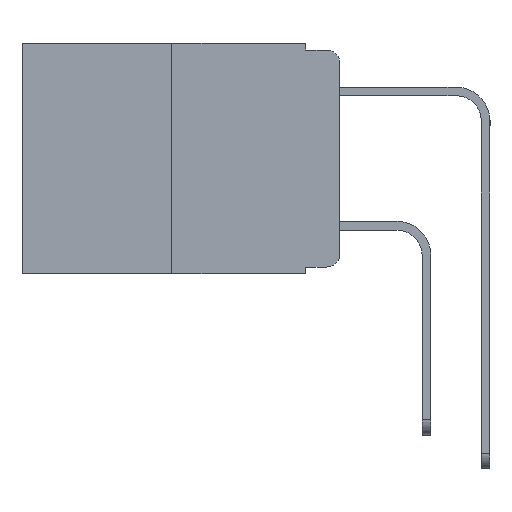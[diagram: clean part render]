
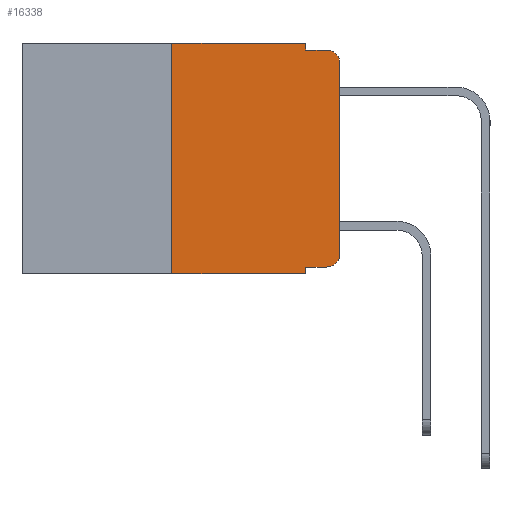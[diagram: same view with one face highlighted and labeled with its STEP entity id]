
A CAD part, left-side view. The second image highlights one B-rep face of the part: STEP entity #16338.
In plain terms, the highlighted planar face has unit normal (-1, 0, 0).
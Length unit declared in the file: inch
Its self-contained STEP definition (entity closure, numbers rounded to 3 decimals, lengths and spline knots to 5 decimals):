
#49 = DIRECTION ( 'NONE',  ( 0., 0., 1. ) ) ;
#77 = CARTESIAN_POINT ( 'NONE',  ( 0., 0.473, 0. ) ) ;
#193 = VERTEX_POINT ( 'NONE', #14427 ) ;
#359 = EDGE_CURVE ( 'NONE', #5972, #6519, #20675, .T. ) ;
#773 = LINE ( 'NONE', #20792, #4306 ) ;
#955 = DIRECTION ( 'NONE',  ( 0., -1., 0. ) ) ;
#1421 = VERTEX_POINT ( 'NONE', #14616 ) ;
#1501 = CARTESIAN_POINT ( 'NONE',  ( 0., 0.02, -0.333 ) ) ;
#1527 = DIRECTION ( 'NONE',  ( -1., 0., 0. ) ) ;
#1548 = EDGE_CURVE ( 'NONE', #13348, #5972, #15921, .T. ) ;
#1756 = DIRECTION ( 'NONE',  ( 0., -1., 0. ) ) ;
#2009 = LINE ( 'NONE', #14542, #18896 ) ;
#2579 = DIRECTION ( 'NONE',  ( 0., 0., 1. ) ) ;
#2585 = CARTESIAN_POINT ( 'NONE',  ( 0., 0., -0.313 ) ) ;
#2716 = EDGE_CURVE ( 'NONE', #13348, #1421, #773, .T. ) ;
#3867 = EDGE_CURVE ( 'NONE', #18301, #6863, #8539, .T. ) ;
#4006 = VECTOR ( 'NONE', #49, 39.37008 ) ;
#4306 = VECTOR ( 'NONE', #13086, 39.37008 ) ;
#4534 = ORIENTED_EDGE ( 'NONE', *, *, #4931, .F. ) ;
#4762 = DIRECTION ( 'NONE',  ( 1., 0., 0. ) ) ;
#4931 = EDGE_CURVE ( 'NONE', #6863, #7960, #19142, .T. ) ;
#5058 = ORIENTED_EDGE ( 'NONE', *, *, #7313, .T. ) ;
#5076 = EDGE_CURVE ( 'NONE', #7960, #16210, #2009, .T. ) ;
#5972 = VERTEX_POINT ( 'NONE', #1501 ) ;
#6217 = EDGE_CURVE ( 'NONE', #16210, #6325, #12436, .T. ) ;
#6325 = VERTEX_POINT ( 'NONE', #10806 ) ;
#6481 = EDGE_LOOP ( 'NONE', ( #16351, #5058, #8260, #9713, #4534, #15453, #9182, #15741, #14504, #7374 ) ) ;
#6519 = VERTEX_POINT ( 'NONE', #2585 ) ;
#6863 = VERTEX_POINT ( 'NONE', #16618 ) ;
#7132 = VECTOR ( 'NONE', #2579, 39.37008 ) ;
#7302 = VECTOR ( 'NONE', #13506, 39.37008 ) ;
#7313 = EDGE_CURVE ( 'NONE', #193, #6325, #11388, .T. ) ;
#7374 = ORIENTED_EDGE ( 'NONE', *, *, #359, .T. ) ;
#7667 = CARTESIAN_POINT ( 'NONE',  ( 0., 0.25, -0.343 ) ) ;
#7801 = CARTESIAN_POINT ( 'NONE',  ( 0., 0.051, -0.01 ) ) ;
#7960 = VERTEX_POINT ( 'NONE', #11371 ) ;
#8084 = PLANE ( 'NONE',  #16501 ) ;
#8260 = ORIENTED_EDGE ( 'NONE', *, *, #6217, .F. ) ;
#8440 = EDGE_CURVE ( 'NONE', #6519, #193, #15763, .T. ) ;
#8539 = LINE ( 'NONE', #14797, #4006 ) ;
#8642 = CARTESIAN_POINT ( 'NONE',  ( 0., 0.02, -0.313 ) ) ;
#9182 = ORIENTED_EDGE ( 'NONE', *, *, #12480, .T. ) ;
#9373 = CARTESIAN_POINT ( 'NONE',  ( 0., 0., 0. ) ) ;
#9713 = ORIENTED_EDGE ( 'NONE', *, *, #5076, .F. ) ;
#9799 = CARTESIAN_POINT ( 'NONE',  ( 0., 0.02, -0.03 ) ) ;
#10315 = VECTOR ( 'NONE', #16185, 39.37008 ) ;
#10806 = CARTESIAN_POINT ( 'NONE',  ( 0., 0.02, -0.01 ) ) ;
#11371 = CARTESIAN_POINT ( 'NONE',  ( 0., 0.051, 0. ) ) ;
#11388 = CIRCLE ( 'NONE', #20933, 0.02 ) ;
#11481 = DIRECTION ( 'NONE',  ( 0., 0., -1. ) ) ;
#12174 = CARTESIAN_POINT ( 'NONE',  ( 0., 0.051, -0.333 ) ) ;
#12436 = LINE ( 'NONE', #13867, #20207 ) ;
#12480 = EDGE_CURVE ( 'NONE', #18301, #1421, #13821, .T. ) ;
#13080 = CARTESIAN_POINT ( 'NONE',  ( 0., 0.473, 0. ) ) ;
#13086 = DIRECTION ( 'NONE',  ( 0., 0., -1. ) ) ;
#13348 = VERTEX_POINT ( 'NONE', #13936 ) ;
#13356 = VECTOR ( 'NONE', #955, 39.37008 ) ;
#13506 = DIRECTION ( 'NONE',  ( 0., -1., 0. ) ) ;
#13821 = LINE ( 'NONE', #20513, #13356 ) ;
#13867 = CARTESIAN_POINT ( 'NONE',  ( 0., 0.051, -0.01 ) ) ;
#13936 = CARTESIAN_POINT ( 'NONE',  ( 0., 0.051, -0.333 ) ) ;
#14427 = CARTESIAN_POINT ( 'NONE',  ( 0., 0., -0.03 ) ) ;
#14504 = ORIENTED_EDGE ( 'NONE', *, *, #1548, .T. ) ;
#14542 = CARTESIAN_POINT ( 'NONE',  ( 0., 0.051, 0. ) ) ;
#14616 = CARTESIAN_POINT ( 'NONE',  ( 0., 0.051, -0.343 ) ) ;
#14797 = CARTESIAN_POINT ( 'NONE',  ( 0., 0.25, 0. ) ) ;
#15279 = DIRECTION ( 'NONE',  ( 0., 0., -1. ) ) ;
#15453 = ORIENTED_EDGE ( 'NONE', *, *, #3867, .F. ) ;
#15741 = ORIENTED_EDGE ( 'NONE', *, *, #2716, .F. ) ;
#15763 = LINE ( 'NONE', #9373, #7132 ) ;
#15921 = LINE ( 'NONE', #12174, #7302 ) ;
#16104 = FACE_OUTER_BOUND ( 'NONE', #6481, .T. ) ;
#16185 = DIRECTION ( 'NONE',  ( 0., -1., 0. ) ) ;
#16204 = DIRECTION ( 'NONE',  ( 0., 0., -1. ) ) ;
#16210 = VERTEX_POINT ( 'NONE', #7801 ) ;
#16338 = ADVANCED_FACE ( 'NONE', ( #16104 ), #8084, .F. ) ;
#16351 = ORIENTED_EDGE ( 'NONE', *, *, #8440, .T. ) ;
#16501 = AXIS2_PLACEMENT_3D ( 'NONE', #13080, #4762, #16204 ) ;
#16618 = CARTESIAN_POINT ( 'NONE',  ( 0., 0.25, 0. ) ) ;
#16968 = AXIS2_PLACEMENT_3D ( 'NONE', #8642, #1527, #15279 ) ;
#18301 = VERTEX_POINT ( 'NONE', #7667 ) ;
#18896 = VECTOR ( 'NONE', #20218, 39.37008 ) ;
#19142 = LINE ( 'NONE', #77, #10315 ) ;
#20207 = VECTOR ( 'NONE', #1756, 39.37008 ) ;
#20218 = DIRECTION ( 'NONE',  ( 0., 0., -1. ) ) ;
#20513 = CARTESIAN_POINT ( 'NONE',  ( 0., 0.473, -0.343 ) ) ;
#20675 = CIRCLE ( 'NONE', #16968, 0.02 ) ;
#20772 = DIRECTION ( 'NONE',  ( -1., 0., 0. ) ) ;
#20792 = CARTESIAN_POINT ( 'NONE',  ( 0., 0.051, 0. ) ) ;
#20933 = AXIS2_PLACEMENT_3D ( 'NONE', #9799, #20772, #11481 ) ;
